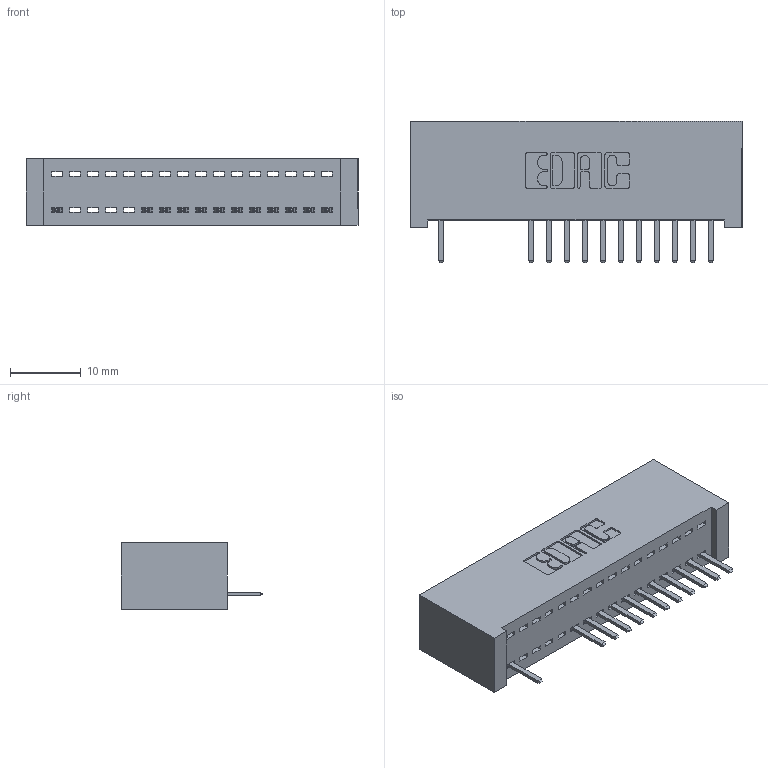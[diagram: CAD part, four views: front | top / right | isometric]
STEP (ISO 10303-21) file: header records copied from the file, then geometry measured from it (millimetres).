
FILE_DESCRIPTION (( 'STEP AP203' ), '1' );
FILE_NAME ('392-016-520-101.STEP', '2018-08-15T01:19:23', ( '' ), ( '' ), 'SwSTEP 2.0', 'SolidWorks 2016', '' );
FILE_SCHEMA (( 'CONFIG_CONTROL_DESIGN' ));
Length unit declared in the file: inch
Products named in the file (3): 342 Part_Lugless; 345-292-001_345-293-120; 392-016-520-101
Assembly tree (13 placements, depth 2):
  392-016-520-101
    342 Part_Lugless
    345-292-001_345-293-120  x12
Bounding box: 46.89 x 20.02 x 9.4 mm (x, y, z)
Volume: 4344.1 mm3; surface area: 5869.5 mm2
Topology: 13 solids, 13 shells, 894 faces, 2651 edges, 1734 vertices
Faces by surface type: plane 638, cylinder 256
Entity records: 12721 total; most frequent: CARTESIAN_POINT 2234, ORIENTED_EDGE 2178, DIRECTION 1913, EDGE_CURVE 1089, LINE 965, VECTOR 965, VERTEX_POINT 722, AXIS2_PLACEMENT_3D 474
